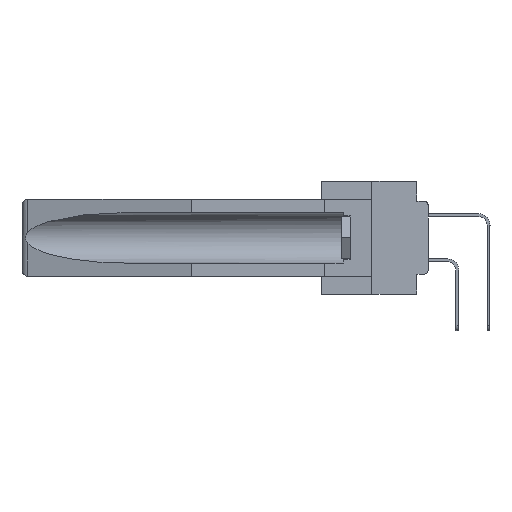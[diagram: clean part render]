
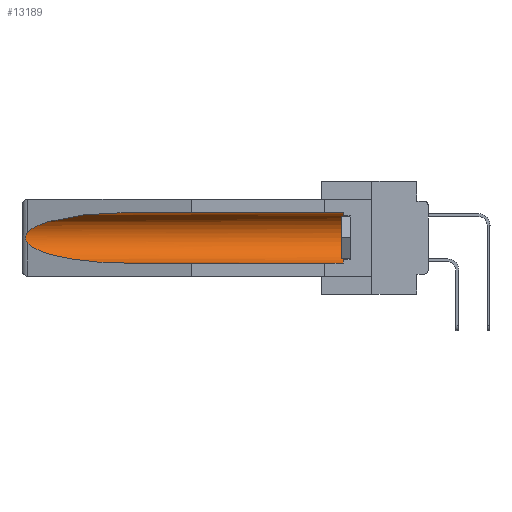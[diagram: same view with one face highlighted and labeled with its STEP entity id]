
A CAD part, left-side view. The second image highlights one B-rep face of the part: STEP entity #13189.
In plain terms, the highlighted cylindrical face has radius 2.857 mm (diameter 5.715 mm), a partial arc.
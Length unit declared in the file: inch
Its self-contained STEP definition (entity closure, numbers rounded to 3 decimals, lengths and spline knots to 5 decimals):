
#468 = FACE_OUTER_BOUND ( 'NONE', #33088, .T. ) ;
#664 = DIRECTION ( 'NONE',  ( 0., 1., 0. ) ) ;
#1044 = DIRECTION ( 'NONE',  ( 0., 0., 1. ) ) ;
#2238 = CARTESIAN_POINT ( 'NONE',  ( 0.26537, 1.52718, -0.19328 ) ) ;
#4719 = AXIS2_PLACEMENT_3D ( 'NONE', #24430, #14472, #1044 ) ;
#4969 = CARTESIAN_POINT ( 'NONE',  ( 0.26597, 1.52961, -0.15275 ) ) ;
#5635 = CARTESIAN_POINT ( 'NONE',  ( 0.155, 1.07973, -0.059 ) ) ;
#5716 = EDGE_CURVE ( 'NONE', #29549, #10313, #23506, .T. ) ;
#5852 = CARTESIAN_POINT ( 'NONE',  ( 0.25451, 1.48313, -0.24835 ) ) ;
#7232 = LINE ( 'NONE', #11744, #16578 ) ;
#7271 = CARTESIAN_POINT ( 'NONE',  ( 0.26537, 1.52718, -0.14972 ) ) ;
#7635 = VERTEX_POINT ( 'NONE', #9208 ) ;
#8008 = CARTESIAN_POINT ( 'NONE',  ( 0.155, 1.07973, -0.284 ) ) ;
#8064 = DIRECTION ( 'NONE',  ( 0., 0., 1. ) ) ;
#8244 =( BOUNDED_CURVE ( )  B_SPLINE_CURVE ( 3, ( #33358, #32906, #17384, #7271 ),
 .UNSPECIFIED., .F., .F. ) 
 B_SPLINE_CURVE_WITH_KNOTS ( ( 4, 4 ),
 ( 4.71239, 6.08839 ),
 .UNSPECIFIED. ) 
 CURVE ( )  GEOMETRIC_REPRESENTATION_ITEM ( )  RATIONAL_B_SPLINE_CURVE ( ( 1., 0.848, 0.848, 1. ) ) 
 REPRESENTATION_ITEM ( '' )  );
#9208 = CARTESIAN_POINT ( 'NONE',  ( 0.26537, 1.52718, -0.14972 ) ) ;
#9749 = LINE ( 'NONE', #21904, #17867 ) ;
#10313 = VERTEX_POINT ( 'NONE', #11596 ) ;
#10564 = ORIENTED_EDGE ( 'NONE', *, *, #27794, .T. ) ;
#11156 = ORIENTED_EDGE ( 'NONE', *, *, #32434, .F. ) ;
#11559 = EDGE_CURVE ( 'NONE', #18105, #30209, #16052, .T. ) ;
#11596 = CARTESIAN_POINT ( 'NONE',  ( 0.155, 1.07973, -0.284 ) ) ;
#11744 = CARTESIAN_POINT ( 'NONE',  ( 0.155, -0.30754, -0.284 ) ) ;
#13189 = ADVANCED_FACE ( 'NONE', ( #468 ), #26048, .F. ) ;
#13849 = CARTESIAN_POINT ( 'NONE',  ( 0.26537, 1.52718, -0.19328 ) ) ;
#14472 = DIRECTION ( 'NONE',  ( 0., -1., 0. ) ) ;
#14828 = CARTESIAN_POINT ( 'NONE',  ( 0.155, 0.126, -0.284 ) ) ;
#14880 = CARTESIAN_POINT ( 'NONE',  ( 0.2673, 1.5327, -0.16383 ) ) ;
#15201 = CARTESIAN_POINT ( 'NONE',  ( 0.26537, 1.52718, -0.14972 ) ) ;
#15315 = CARTESIAN_POINT ( 'NONE',  ( 0.2675, 1.53308, -0.16763 ) ) ;
#16052 = CIRCLE ( 'NONE', #4719, 0.1125 ) ;
#16578 = VECTOR ( 'NONE', #19560, 39.37008 ) ;
#16839 = CARTESIAN_POINT ( 'NONE',  ( 0.155, 0.126, -0.059 ) ) ;
#17384 = CARTESIAN_POINT ( 'NONE',  ( 0.25451, 1.48313, -0.09465 ) ) ;
#17867 = VECTOR ( 'NONE', #664, 39.37008 ) ;
#18105 = VERTEX_POINT ( 'NONE', #14828 ) ;
#19106 = ORIENTED_EDGE ( 'NONE', *, *, #5716, .T. ) ;
#19560 = DIRECTION ( 'NONE',  ( 0., 1., 0. ) ) ;
#20238 = EDGE_CURVE ( 'NONE', #30209, #28143, #9749, .T. ) ;
#20408 = CARTESIAN_POINT ( 'NONE',  ( 0.26597, 1.5296, -0.19026 ) ) ;
#20977 = CARTESIAN_POINT ( 'NONE',  ( 0.21114, 1.30732, -0.284 ) ) ;
#21904 = CARTESIAN_POINT ( 'NONE',  ( 0.155, -0.30754, -0.059 ) ) ;
#23506 =( BOUNDED_CURVE ( )  B_SPLINE_CURVE ( 3, ( #23581, #5852, #20977, #8008 ),
 .UNSPECIFIED., .F., .F. ) 
 B_SPLINE_CURVE_WITH_KNOTS ( ( 4, 4 ),
 ( 0.1948, 1.5708 ),
 .UNSPECIFIED. ) 
 CURVE ( )  GEOMETRIC_REPRESENTATION_ITEM ( )  RATIONAL_B_SPLINE_CURVE ( ( 1., 0.848, 0.848, 1. ) ) 
 REPRESENTATION_ITEM ( '' )  );
#23581 = CARTESIAN_POINT ( 'NONE',  ( 0.26537, 1.52718, -0.19328 ) ) ;
#23639 = CARTESIAN_POINT ( 'NONE',  ( 0.155, -0.30754, -0.1715 ) ) ;
#23961 = DIRECTION ( 'NONE',  ( 0., 1., 0. ) ) ;
#24430 = CARTESIAN_POINT ( 'NONE',  ( 0.155, 0.126, -0.1715 ) ) ;
#25521 = ORIENTED_EDGE ( 'NONE', *, *, #11559, .T. ) ;
#26048 = CYLINDRICAL_SURFACE ( 'NONE', #29289, 0.1125 ) ;
#26778 = EDGE_CURVE ( 'NONE', #28143, #7635, #8244, .T. ) ;
#26961 = B_SPLINE_CURVE_WITH_KNOTS ( 'NONE', 3,
 ( #15201, #4969, #30816, #14880, #15315, #33423, #30597, #27995, #20408, #2238 ),
 .UNSPECIFIED., .F., .F.,
 ( 4, 2, 2, 2, 4 ),
 ( 0., 0.00029, 0.00058, 0.00087, 0.00117 ),
 .UNSPECIFIED. ) ;
#27794 = EDGE_CURVE ( 'NONE', #7635, #29549, #26961, .T. ) ;
#27995 = CARTESIAN_POINT ( 'NONE',  ( 0.26655, 1.53094, -0.18657 ) ) ;
#28143 = VERTEX_POINT ( 'NONE', #5635 ) ;
#29289 = AXIS2_PLACEMENT_3D ( 'NONE', #23639, #23961, #8064 ) ;
#29549 = VERTEX_POINT ( 'NONE', #13849 ) ;
#30209 = VERTEX_POINT ( 'NONE', #16839 ) ;
#30597 = CARTESIAN_POINT ( 'NONE',  ( 0.2673, 1.53269, -0.17917 ) ) ;
#30816 = CARTESIAN_POINT ( 'NONE',  ( 0.26654, 1.53092, -0.15636 ) ) ;
#32434 = EDGE_CURVE ( 'NONE', #18105, #10313, #7232, .T. ) ;
#32906 = CARTESIAN_POINT ( 'NONE',  ( 0.21114, 1.30732, -0.059 ) ) ;
#33012 = ORIENTED_EDGE ( 'NONE', *, *, #20238, .T. ) ;
#33088 = EDGE_LOOP ( 'NONE', ( #33213, #10564, #19106, #11156, #25521, #33012 ) ) ;
#33213 = ORIENTED_EDGE ( 'NONE', *, *, #26778, .T. ) ;
#33358 = CARTESIAN_POINT ( 'NONE',  ( 0.155, 1.07973, -0.059 ) ) ;
#33423 = CARTESIAN_POINT ( 'NONE',  ( 0.2675, 1.53308, -0.17534 ) ) ;
